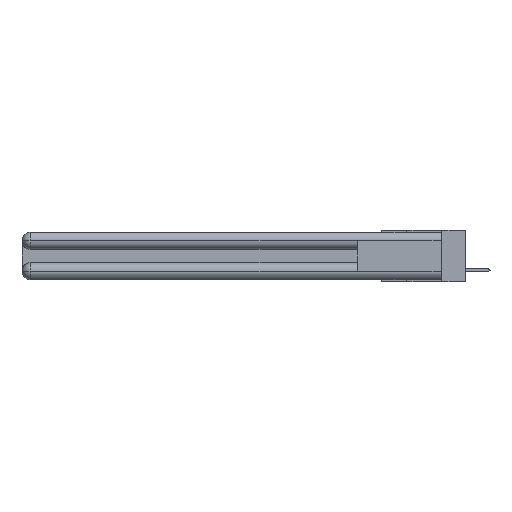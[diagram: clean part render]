
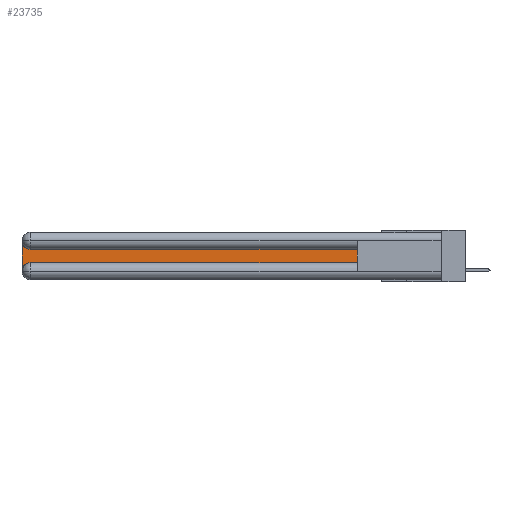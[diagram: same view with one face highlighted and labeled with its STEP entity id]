
A CAD part, left-side view. The second image highlights one B-rep face of the part: STEP entity #23735.
In plain terms, the highlighted planar face has unit normal (-1, 0, 0).
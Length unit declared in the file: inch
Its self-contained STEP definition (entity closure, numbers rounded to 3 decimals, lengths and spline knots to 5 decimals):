
#606 = CARTESIAN_POINT ( 'NONE',  ( 0.075, 2.94, -0.2175 ) ) ;
#959 = DIRECTION ( 'NONE',  ( 0., 0., 1. ) ) ;
#2216 = EDGE_LOOP ( 'NONE', ( #18548, #2567, #25171, #12503, #10915, #4516 ) ) ;
#2567 = ORIENTED_EDGE ( 'NONE', *, *, #3019, .T. ) ;
#2634 = VERTEX_POINT ( 'NONE', #22853 ) ;
#2743 = CARTESIAN_POINT ( 'NONE',  ( 0.075, 0.6, -0.1225 ) ) ;
#2906 = CARTESIAN_POINT ( 'NONE',  ( 0.075, 0.6, -0.2175 ) ) ;
#2936 = VECTOR ( 'NONE', #11190, 39.37008 ) ;
#3019 = EDGE_CURVE ( 'NONE', #13946, #23723, #12160, .T. ) ;
#4077 = VECTOR ( 'NONE', #21399, 39.37008 ) ;
#4516 = ORIENTED_EDGE ( 'NONE', *, *, #16760, .T. ) ;
#5568 = VERTEX_POINT ( 'NONE', #6772 ) ;
#5781 = EDGE_CURVE ( 'NONE', #15922, #5568, #18765, .T. ) ;
#6033 = LINE ( 'NONE', #2743, #4077 ) ;
#6772 = CARTESIAN_POINT ( 'NONE',  ( 0.075, 0.6, -0.2175 ) ) ;
#7189 = CARTESIAN_POINT ( 'NONE',  ( 0.075, 0.6, -0.1225 ) ) ;
#7476 = EDGE_CURVE ( 'NONE', #2634, #15922, #8985, .T. ) ;
#7569 = DIRECTION ( 'NONE',  ( 1., 0., 0. ) ) ;
#7596 = AXIS2_PLACEMENT_3D ( 'NONE', #18330, #7569, #22364 ) ;
#7607 = DIRECTION ( 'NONE',  ( 1., 0., 0. ) ) ;
#8176 = LINE ( 'NONE', #19424, #23356 ) ;
#8985 = CIRCLE ( 'NONE', #9907, 0.06 ) ;
#9767 = CARTESIAN_POINT ( 'NONE',  ( 0.075, 3., -0.1225 ) ) ;
#9907 = AXIS2_PLACEMENT_3D ( 'NONE', #22330, #20076, #20155 ) ;
#10915 = ORIENTED_EDGE ( 'NONE', *, *, #5781, .T. ) ;
#11190 = DIRECTION ( 'NONE',  ( 0., -1., 0. ) ) ;
#11860 = DIRECTION ( 'NONE',  ( 0., 0., -1. ) ) ;
#12160 = CIRCLE ( 'NONE', #7596, 0.06 ) ;
#12322 = CARTESIAN_POINT ( 'NONE',  ( 0.075, 2.94, -0.1225 ) ) ;
#12503 = ORIENTED_EDGE ( 'NONE', *, *, #7476, .T. ) ;
#12841 = CARTESIAN_POINT ( 'NONE',  ( 0.075, 3., -0.2175 ) ) ;
#13765 = CARTESIAN_POINT ( 'NONE',  ( 0.075, 3., -0.0625 ) ) ;
#13946 = VERTEX_POINT ( 'NONE', #12322 ) ;
#14088 = EDGE_CURVE ( 'NONE', #23723, #2634, #20547, .T. ) ;
#14094 = EDGE_CURVE ( 'NONE', #15772, #13946, #6033, .T. ) ;
#15071 = VECTOR ( 'NONE', #19069, 39.37008 ) ;
#15772 = VERTEX_POINT ( 'NONE', #7189 ) ;
#15922 = VERTEX_POINT ( 'NONE', #606 ) ;
#16760 = EDGE_CURVE ( 'NONE', #5568, #15772, #8176, .T. ) ;
#18330 = CARTESIAN_POINT ( 'NONE',  ( 0.075, 2.94, -0.0625 ) ) ;
#18548 = ORIENTED_EDGE ( 'NONE', *, *, #14094, .T. ) ;
#18765 = LINE ( 'NONE', #2906, #2936 ) ;
#19069 = DIRECTION ( 'NONE',  ( 0., 0., -1. ) ) ;
#19424 = CARTESIAN_POINT ( 'NONE',  ( 0.075, 0.6, -0.2175 ) ) ;
#20076 = DIRECTION ( 'NONE',  ( 1., 0., 0. ) ) ;
#20155 = DIRECTION ( 'NONE',  ( 0., 0., -1. ) ) ;
#20547 = LINE ( 'NONE', #12841, #15071 ) ;
#21399 = DIRECTION ( 'NONE',  ( 0., 1., 0. ) ) ;
#22330 = CARTESIAN_POINT ( 'NONE',  ( 0.075, 2.94, -0.2775 ) ) ;
#22364 = DIRECTION ( 'NONE',  ( 0., 0., -1. ) ) ;
#22784 = AXIS2_PLACEMENT_3D ( 'NONE', #9767, #7607, #11860 ) ;
#22853 = CARTESIAN_POINT ( 'NONE',  ( 0.075, 3., -0.2775 ) ) ;
#23304 = FACE_OUTER_BOUND ( 'NONE', #2216, .T. ) ;
#23356 = VECTOR ( 'NONE', #959, 39.37008 ) ;
#23723 = VERTEX_POINT ( 'NONE', #13765 ) ;
#23735 = ADVANCED_FACE ( 'NONE', ( #23304 ), #24027, .F. ) ;
#24027 = PLANE ( 'NONE',  #22784 ) ;
#25171 = ORIENTED_EDGE ( 'NONE', *, *, #14088, .T. ) ;
